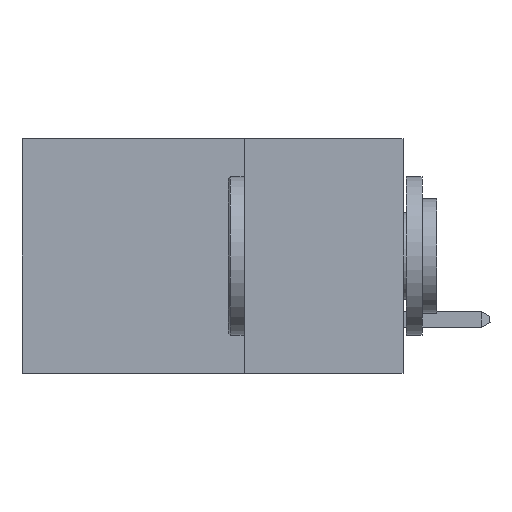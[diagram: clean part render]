
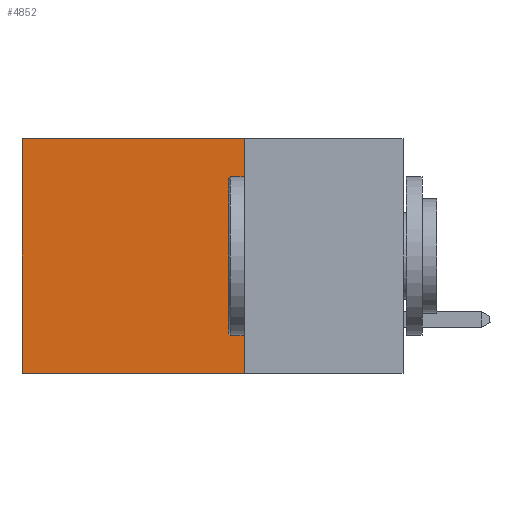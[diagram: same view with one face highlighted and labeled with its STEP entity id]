
A CAD part, left-side view. The second image highlights one B-rep face of the part: STEP entity #4852.
In plain terms, the highlighted planar face has unit normal (-1, 0, 0).
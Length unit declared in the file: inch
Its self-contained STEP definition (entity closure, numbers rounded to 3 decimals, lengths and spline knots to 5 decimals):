
#2885 = CARTESIAN_POINT ( 'NONE',  ( 0.2875, 0.25, -0.37 ) ) ;
#3549 = CARTESIAN_POINT ( 'NONE',  ( 0.2875, 0.6, 0. ) ) ;
#3839 = VERTEX_POINT ( 'NONE', #2885 ) ;
#4852 = ADVANCED_FACE ( 'NONE', ( #38289 ), #25799, .F. ) ;
#5240 = VECTOR ( 'NONE', #15548, 39.37008 ) ;
#6598 = DIRECTION ( 'NONE',  ( 0., 0., -1. ) ) ;
#6914 = CARTESIAN_POINT ( 'NONE',  ( 0.2875, 0.25, 0. ) ) ;
#7017 = VECTOR ( 'NONE', #35652, 39.37008 ) ;
#7155 = DIRECTION ( 'NONE',  ( 0., 1., 0. ) ) ;
#7795 = CARTESIAN_POINT ( 'NONE',  ( 0.2875, 0.25, 0. ) ) ;
#8360 = VECTOR ( 'NONE', #7155, 39.37008 ) ;
#10837 = DIRECTION ( 'NONE',  ( 1., 0., 0. ) ) ;
#13297 = EDGE_CURVE ( 'NONE', #23933, #30822, #25283, .T. ) ;
#13870 = CARTESIAN_POINT ( 'NONE',  ( 0.2875, 0.6, -0.37 ) ) ;
#15548 = DIRECTION ( 'NONE',  ( 0., 0., -1. ) ) ;
#17651 = ORIENTED_EDGE ( 'NONE', *, *, #38152, .T. ) ;
#21172 = LINE ( 'NONE', #3549, #37232 ) ;
#21249 = LINE ( 'NONE', #27533, #5240 ) ;
#23599 = CARTESIAN_POINT ( 'NONE',  ( 0.2875, 0.6, 0. ) ) ;
#23933 = VERTEX_POINT ( 'NONE', #6914 ) ;
#24410 = ORIENTED_EDGE ( 'NONE', *, *, #24527, .F. ) ;
#24527 = EDGE_CURVE ( 'NONE', #23933, #3839, #21249, .T. ) ;
#24882 = LINE ( 'NONE', #29553, #7017 ) ;
#25283 = LINE ( 'NONE', #31260, #8360 ) ;
#25477 = ORIENTED_EDGE ( 'NONE', *, *, #13297, .T. ) ;
#25739 = EDGE_CURVE ( 'NONE', #3839, #28804, #24882, .T. ) ;
#25799 = PLANE ( 'NONE',  #34619 ) ;
#27533 = CARTESIAN_POINT ( 'NONE',  ( 0.2875, 0.25, 0. ) ) ;
#28804 = VERTEX_POINT ( 'NONE', #13870 ) ;
#29553 = CARTESIAN_POINT ( 'NONE',  ( 0.2875, 0.25, -0.37 ) ) ;
#30822 = VERTEX_POINT ( 'NONE', #23599 ) ;
#31260 = CARTESIAN_POINT ( 'NONE',  ( 0.2875, 0.25, 0. ) ) ;
#31915 = DIRECTION ( 'NONE',  ( 0., 0., -1. ) ) ;
#33828 = ORIENTED_EDGE ( 'NONE', *, *, #25739, .F. ) ;
#34619 = AXIS2_PLACEMENT_3D ( 'NONE', #7795, #10837, #31915 ) ;
#35652 = DIRECTION ( 'NONE',  ( 0., 1., 0. ) ) ;
#37232 = VECTOR ( 'NONE', #6598, 39.37008 ) ;
#38081 = EDGE_LOOP ( 'NONE', ( #17651, #33828, #24410, #25477 ) ) ;
#38152 = EDGE_CURVE ( 'NONE', #30822, #28804, #21172, .T. ) ;
#38289 = FACE_OUTER_BOUND ( 'NONE', #38081, .T. ) ;
